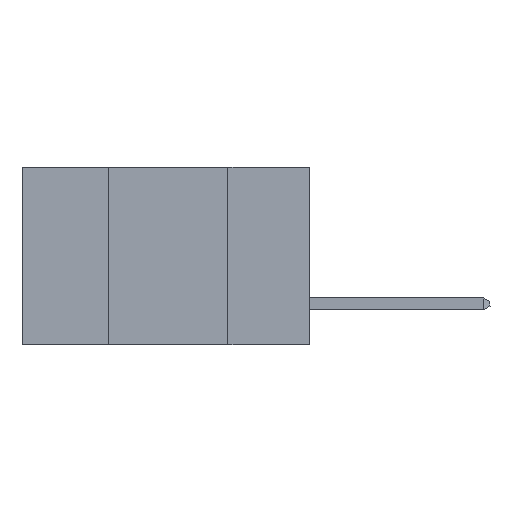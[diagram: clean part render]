
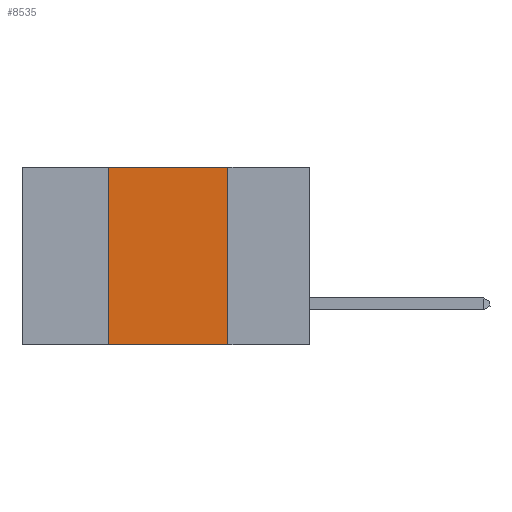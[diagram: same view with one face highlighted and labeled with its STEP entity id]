
A CAD part, left-side view. The second image highlights one B-rep face of the part: STEP entity #8535.
In plain terms, the highlighted planar face has unit normal (-1, 0, 0).
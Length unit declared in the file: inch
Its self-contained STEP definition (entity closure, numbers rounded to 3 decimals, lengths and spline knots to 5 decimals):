
#158 = EDGE_CURVE ( 'NONE', #7092, #8173, #10934, .T. ) ;
#387 = ORIENTED_EDGE ( 'NONE', *, *, #6706, .F. ) ;
#477 = CARTESIAN_POINT ( 'NONE',  ( 0., 0.6, 0. ) ) ;
#693 = ORIENTED_EDGE ( 'NONE', *, *, #158, .F. ) ;
#1052 = CARTESIAN_POINT ( 'NONE',  ( 0., 0.17, 0. ) ) ;
#2284 = DIRECTION ( 'NONE',  ( 0., 0., -1. ) ) ;
#3161 = PLANE ( 'NONE',  #10402 ) ;
#3169 = EDGE_CURVE ( 'NONE', #9365, #6404, #3839, .T. ) ;
#3292 = FACE_OUTER_BOUND ( 'NONE', #8830, .T. ) ;
#3376 = VECTOR ( 'NONE', #2284, 39.37008 ) ;
#3483 = CARTESIAN_POINT ( 'NONE',  ( 0., 0.17, -0.37 ) ) ;
#3572 = DIRECTION ( 'NONE',  ( 0., -1., 0. ) ) ;
#3809 = DIRECTION ( 'NONE',  ( 0., 0., 1. ) ) ;
#3839 = LINE ( 'NONE', #9492, #5928 ) ;
#4113 = ORIENTED_EDGE ( 'NONE', *, *, #3169, .F. ) ;
#4140 = CARTESIAN_POINT ( 'NONE',  ( 0., 0.6, 0. ) ) ;
#4517 = ORIENTED_EDGE ( 'NONE', *, *, #10566, .T. ) ;
#5090 = VECTOR ( 'NONE', #10646, 39.37008 ) ;
#5928 = VECTOR ( 'NONE', #3809, 39.37008 ) ;
#5983 = LINE ( 'NONE', #4140, #5090 ) ;
#6404 = VERTEX_POINT ( 'NONE', #7580 ) ;
#6706 = EDGE_CURVE ( 'NONE', #6404, #7092, #5983, .T. ) ;
#7029 = VECTOR ( 'NONE', #3572, 39.37008 ) ;
#7092 = VERTEX_POINT ( 'NONE', #1052 ) ;
#7580 = CARTESIAN_POINT ( 'NONE',  ( 0., 0.42, 0. ) ) ;
#7665 = CARTESIAN_POINT ( 'NONE',  ( 0., 0.17, 0. ) ) ;
#8173 = VERTEX_POINT ( 'NONE', #3483 ) ;
#8535 = ADVANCED_FACE ( 'NONE', ( #3292 ), #3161, .F. ) ;
#8830 = EDGE_LOOP ( 'NONE', ( #693, #387, #4113, #4517 ) ) ;
#9130 = CARTESIAN_POINT ( 'NONE',  ( 0., 0.6, -0.37 ) ) ;
#9365 = VERTEX_POINT ( 'NONE', #10244 ) ;
#9492 = CARTESIAN_POINT ( 'NONE',  ( 0., 0.42, 0. ) ) ;
#9646 = DIRECTION ( 'NONE',  ( 0., 0., -1. ) ) ;
#10244 = CARTESIAN_POINT ( 'NONE',  ( 0., 0.42, -0.37 ) ) ;
#10402 = AXIS2_PLACEMENT_3D ( 'NONE', #477, #10509, #9646 ) ;
#10509 = DIRECTION ( 'NONE',  ( 1., 0., 0. ) ) ;
#10512 = LINE ( 'NONE', #9130, #7029 ) ;
#10566 = EDGE_CURVE ( 'NONE', #9365, #8173, #10512, .T. ) ;
#10646 = DIRECTION ( 'NONE',  ( 0., -1., 0. ) ) ;
#10934 = LINE ( 'NONE', #7665, #3376 ) ;
